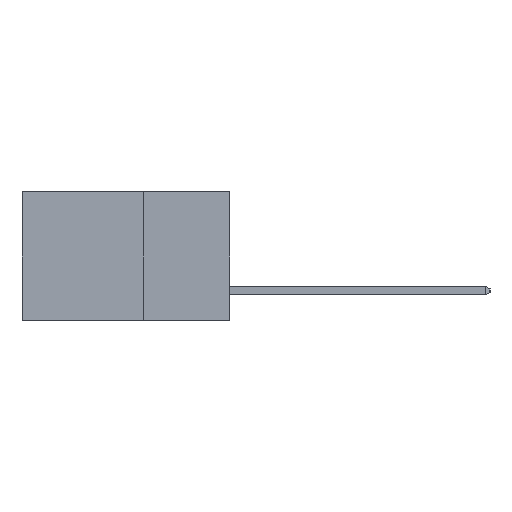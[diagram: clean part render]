
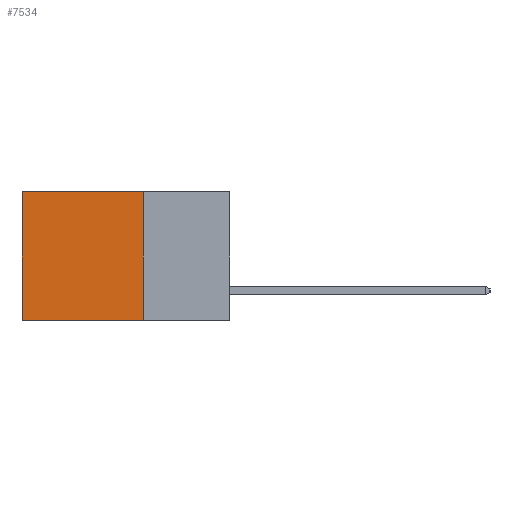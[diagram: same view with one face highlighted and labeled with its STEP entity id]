
A CAD part, left-side view. The second image highlights one B-rep face of the part: STEP entity #7534.
In plain terms, the highlighted planar face has unit normal (-1, 0, 0).
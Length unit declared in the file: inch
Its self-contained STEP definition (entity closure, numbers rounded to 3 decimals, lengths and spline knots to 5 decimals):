
#147 = ORIENTED_EDGE ( 'NONE', *, *, #7051, .T. ) ;
#858 = LINE ( 'NONE', #4840, #16256 ) ;
#1267 = VERTEX_POINT ( 'NONE', #15665 ) ;
#1646 = CARTESIAN_POINT ( 'NONE',  ( 0.2615, 0.6, 0. ) ) ;
#1739 = ORIENTED_EDGE ( 'NONE', *, *, #8503, .T. ) ;
#1765 = VECTOR ( 'NONE', #17987, 39.37008 ) ;
#2657 = CARTESIAN_POINT ( 'NONE',  ( 0.2615, 0.25, -0.37 ) ) ;
#2683 = DIRECTION ( 'NONE',  ( 0., 1., 0. ) ) ;
#3002 = ORIENTED_EDGE ( 'NONE', *, *, #13910, .F. ) ;
#3884 = CARTESIAN_POINT ( 'NONE',  ( 0.2615, 0.6, -0.37 ) ) ;
#4393 = LINE ( 'NONE', #4828, #1765 ) ;
#4534 = DIRECTION ( 'NONE',  ( 0., 0., -1. ) ) ;
#4828 = CARTESIAN_POINT ( 'NONE',  ( 0.2615, 0.25, -0.37 ) ) ;
#4840 = CARTESIAN_POINT ( 'NONE',  ( 0.2615, 0.6, -0.37 ) ) ;
#5001 = AXIS2_PLACEMENT_3D ( 'NONE', #8871, #8268, #8214 ) ;
#6384 = EDGE_LOOP ( 'NONE', ( #147, #14113, #3002, #1739 ) ) ;
#6510 = LINE ( 'NONE', #12100, #17731 ) ;
#7051 = EDGE_CURVE ( 'NONE', #11471, #9260, #858, .T. ) ;
#7156 = EDGE_CURVE ( 'NONE', #8702, #9260, #18679, .T. ) ;
#7534 = ADVANCED_FACE ( 'NONE', ( #16242 ), #8509, .F. ) ;
#8214 = DIRECTION ( 'NONE',  ( 0., 0., -1. ) ) ;
#8268 = DIRECTION ( 'NONE',  ( 1., 0., 0. ) ) ;
#8503 = EDGE_CURVE ( 'NONE', #1267, #11471, #6510, .T. ) ;
#8509 = PLANE ( 'NONE',  #5001 ) ;
#8702 = VERTEX_POINT ( 'NONE', #10198 ) ;
#8871 = CARTESIAN_POINT ( 'NONE',  ( 0.2615, 0.25, -0.37 ) ) ;
#9260 = VERTEX_POINT ( 'NONE', #3884 ) ;
#10198 = CARTESIAN_POINT ( 'NONE',  ( 0.2615, 0.25, -0.37 ) ) ;
#11003 = VECTOR ( 'NONE', #2683, 39.37008 ) ;
#11471 = VERTEX_POINT ( 'NONE', #1646 ) ;
#12100 = CARTESIAN_POINT ( 'NONE',  ( 0.2615, 0.25, 0. ) ) ;
#12359 = DIRECTION ( 'NONE',  ( 0., 1., 0. ) ) ;
#13910 = EDGE_CURVE ( 'NONE', #1267, #8702, #4393, .T. ) ;
#14113 = ORIENTED_EDGE ( 'NONE', *, *, #7156, .F. ) ;
#15665 = CARTESIAN_POINT ( 'NONE',  ( 0.2615, 0.25, 0. ) ) ;
#16242 = FACE_OUTER_BOUND ( 'NONE', #6384, .T. ) ;
#16256 = VECTOR ( 'NONE', #4534, 39.37008 ) ;
#17731 = VECTOR ( 'NONE', #12359, 39.37008 ) ;
#17987 = DIRECTION ( 'NONE',  ( 0., 0., -1. ) ) ;
#18679 = LINE ( 'NONE', #2657, #11003 ) ;
